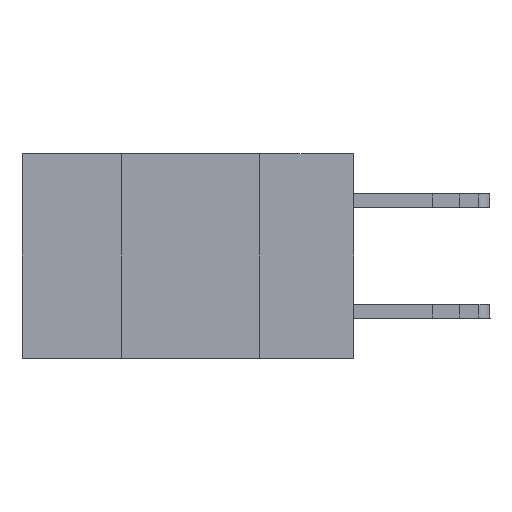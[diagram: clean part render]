
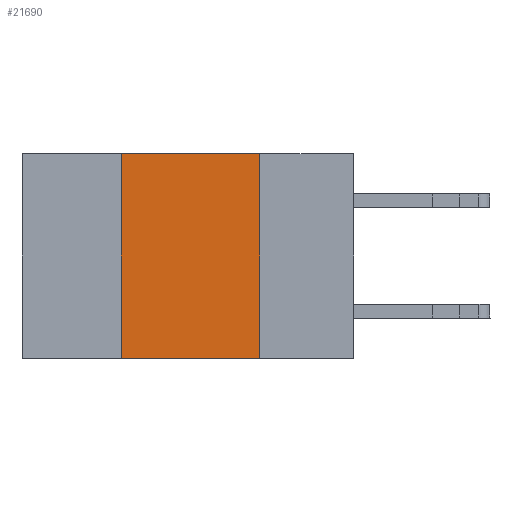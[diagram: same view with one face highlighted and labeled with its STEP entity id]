
A CAD part, left-side view. The second image highlights one B-rep face of the part: STEP entity #21690.
In plain terms, the highlighted planar face has unit normal (-1, 0, 0).
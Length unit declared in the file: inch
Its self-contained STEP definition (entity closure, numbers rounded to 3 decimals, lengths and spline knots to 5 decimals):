
#2306 = ORIENTED_EDGE ( 'NONE', *, *, #21156, .F. ) ;
#2533 = ORIENTED_EDGE ( 'NONE', *, *, #13480, .T. ) ;
#3165 = FACE_OUTER_BOUND ( 'NONE', #11951, .T. ) ;
#3269 = CARTESIAN_POINT ( 'NONE',  ( 0., 0.42, 0. ) ) ;
#4676 = CARTESIAN_POINT ( 'NONE',  ( 0., 0.6, 0. ) ) ;
#4812 = PLANE ( 'NONE',  #14275 ) ;
#4911 = LINE ( 'NONE', #6438, #7917 ) ;
#6282 = VECTOR ( 'NONE', #6686, 39.37008 ) ;
#6438 = CARTESIAN_POINT ( 'NONE',  ( 0., 0.6, -0.37 ) ) ;
#6576 = DIRECTION ( 'NONE',  ( 1., 0., 0. ) ) ;
#6686 = DIRECTION ( 'NONE',  ( 0., 0., 1. ) ) ;
#6780 = DIRECTION ( 'NONE',  ( 0., -1., 0. ) ) ;
#7320 = DIRECTION ( 'NONE',  ( 0., 0., -1. ) ) ;
#7917 = VECTOR ( 'NONE', #6780, 39.37008 ) ;
#8503 = CARTESIAN_POINT ( 'NONE',  ( 0., 0.6, 0. ) ) ;
#8790 = ORIENTED_EDGE ( 'NONE', *, *, #12432, .F. ) ;
#11951 = EDGE_LOOP ( 'NONE', ( #8790, #14540, #2306, #2533 ) ) ;
#12253 = CARTESIAN_POINT ( 'NONE',  ( 0., 0.17, 0. ) ) ;
#12432 = EDGE_CURVE ( 'NONE', #13462, #12520, #14456, .T. ) ;
#12520 = VERTEX_POINT ( 'NONE', #21560 ) ;
#13462 = VERTEX_POINT ( 'NONE', #12253 ) ;
#13480 = EDGE_CURVE ( 'NONE', #21465, #12520, #4911, .T. ) ;
#14275 = AXIS2_PLACEMENT_3D ( 'NONE', #8503, #6576, #19418 ) ;
#14456 = LINE ( 'NONE', #15972, #22507 ) ;
#14540 = ORIENTED_EDGE ( 'NONE', *, *, #21298, .F. ) ;
#15899 = CARTESIAN_POINT ( 'NONE',  ( 0., 0.42, -0.37 ) ) ;
#15972 = CARTESIAN_POINT ( 'NONE',  ( 0., 0.17, 0. ) ) ;
#19418 = DIRECTION ( 'NONE',  ( 0., 0., -1. ) ) ;
#19422 = CARTESIAN_POINT ( 'NONE',  ( 0., 0.42, 0. ) ) ;
#19648 = LINE ( 'NONE', #19422, #6282 ) ;
#21156 = EDGE_CURVE ( 'NONE', #21465, #21706, #19648, .T. ) ;
#21298 = EDGE_CURVE ( 'NONE', #21706, #13462, #22335, .T. ) ;
#21465 = VERTEX_POINT ( 'NONE', #15899 ) ;
#21560 = CARTESIAN_POINT ( 'NONE',  ( 0., 0.17, -0.37 ) ) ;
#21690 = ADVANCED_FACE ( 'NONE', ( #3165 ), #4812, .F. ) ;
#21706 = VERTEX_POINT ( 'NONE', #3269 ) ;
#22335 = LINE ( 'NONE', #4676, #23211 ) ;
#22507 = VECTOR ( 'NONE', #7320, 39.37008 ) ;
#22577 = DIRECTION ( 'NONE',  ( 0., -1., 0. ) ) ;
#23211 = VECTOR ( 'NONE', #22577, 39.37008 ) ;
